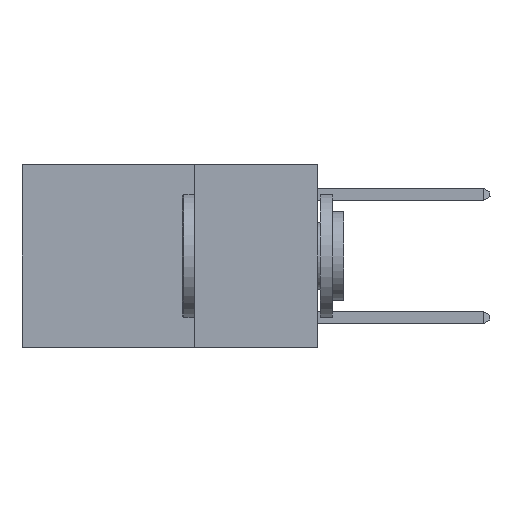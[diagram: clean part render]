
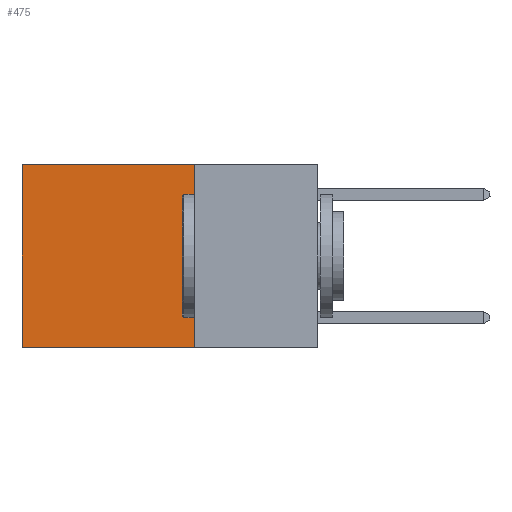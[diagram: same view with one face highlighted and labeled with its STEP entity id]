
A CAD part, left-side view. The second image highlights one B-rep face of the part: STEP entity #475.
In plain terms, the highlighted planar face has unit normal (-1, 0, 0).
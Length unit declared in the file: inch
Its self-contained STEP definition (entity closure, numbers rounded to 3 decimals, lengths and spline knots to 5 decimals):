
#228 = CARTESIAN_POINT ( 'NONE',  ( 0.2625, 0.25, 0. ) ) ;
#475 = ADVANCED_FACE ( 'NONE', ( #14536 ), #14833, .F. ) ;
#697 = LINE ( 'NONE', #12187, #13888 ) ;
#1490 = DIRECTION ( 'NONE',  ( 0., 0., -1. ) ) ;
#2192 = ORIENTED_EDGE ( 'NONE', *, *, #13976, .F. ) ;
#2822 = VERTEX_POINT ( 'NONE', #14434 ) ;
#3182 = EDGE_CURVE ( 'NONE', #2822, #8188, #697, .T. ) ;
#4000 = ORIENTED_EDGE ( 'NONE', *, *, #5133, .F. ) ;
#4262 = DIRECTION ( 'NONE',  ( 0., 0., -1. ) ) ;
#5133 = EDGE_CURVE ( 'NONE', #11441, #8188, #13143, .T. ) ;
#5374 = VECTOR ( 'NONE', #4262, 39.37008 ) ;
#5726 = CARTESIAN_POINT ( 'NONE',  ( 0.2625, 0.25, -0.37 ) ) ;
#6150 = DIRECTION ( 'NONE',  ( 0., 1., 0. ) ) ;
#7008 = EDGE_LOOP ( 'NONE', ( #9801, #4000, #2192, #17927 ) ) ;
#7226 = CARTESIAN_POINT ( 'NONE',  ( 0.2625, 0.25, 0. ) ) ;
#7785 = DIRECTION ( 'NONE',  ( 0., 0., -1. ) ) ;
#8188 = VERTEX_POINT ( 'NONE', #17147 ) ;
#8524 = CARTESIAN_POINT ( 'NONE',  ( 0.2625, 0.25, 0. ) ) ;
#9801 = ORIENTED_EDGE ( 'NONE', *, *, #3182, .T. ) ;
#10202 = DIRECTION ( 'NONE',  ( 0., 1., 0. ) ) ;
#10258 = VECTOR ( 'NONE', #10202, 39.37008 ) ;
#11434 = EDGE_CURVE ( 'NONE', #18386, #2822, #13573, .T. ) ;
#11441 = VERTEX_POINT ( 'NONE', #13203 ) ;
#11677 = LINE ( 'NONE', #17619, #5374 ) ;
#12187 = CARTESIAN_POINT ( 'NONE',  ( 0.2625, 0.6, 0. ) ) ;
#13139 = VECTOR ( 'NONE', #6150, 39.37008 ) ;
#13143 = LINE ( 'NONE', #5726, #10258 ) ;
#13203 = CARTESIAN_POINT ( 'NONE',  ( 0.2625, 0.25, -0.37 ) ) ;
#13573 = LINE ( 'NONE', #228, #13139 ) ;
#13888 = VECTOR ( 'NONE', #7785, 39.37008 ) ;
#13976 = EDGE_CURVE ( 'NONE', #18386, #11441, #11677, .T. ) ;
#14183 = AXIS2_PLACEMENT_3D ( 'NONE', #7226, #19175, #1490 ) ;
#14434 = CARTESIAN_POINT ( 'NONE',  ( 0.2625, 0.6, 0. ) ) ;
#14536 = FACE_OUTER_BOUND ( 'NONE', #7008, .T. ) ;
#14833 = PLANE ( 'NONE',  #14183 ) ;
#17147 = CARTESIAN_POINT ( 'NONE',  ( 0.2625, 0.6, -0.37 ) ) ;
#17619 = CARTESIAN_POINT ( 'NONE',  ( 0.2625, 0.25, 0. ) ) ;
#17927 = ORIENTED_EDGE ( 'NONE', *, *, #11434, .T. ) ;
#18386 = VERTEX_POINT ( 'NONE', #8524 ) ;
#19175 = DIRECTION ( 'NONE',  ( 1., 0., 0. ) ) ;
